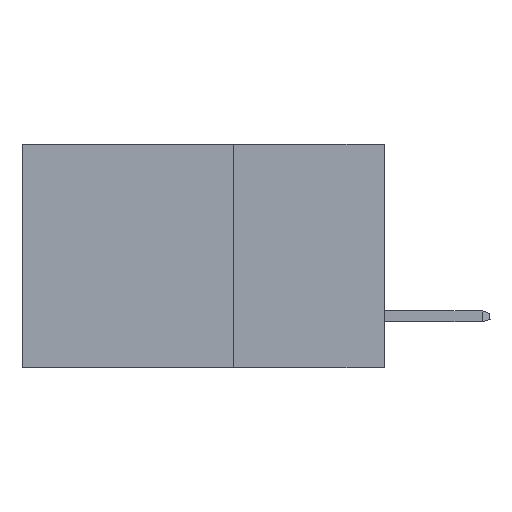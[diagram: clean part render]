
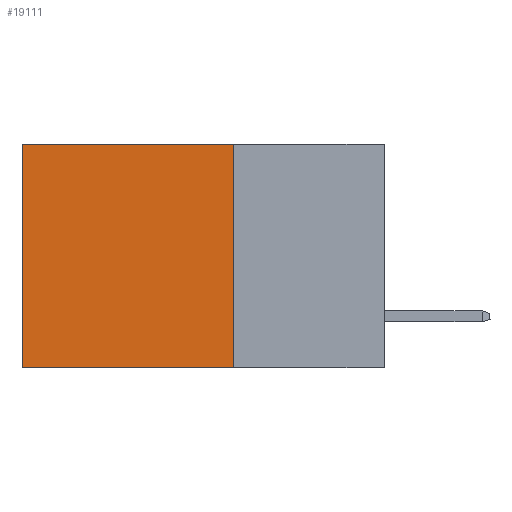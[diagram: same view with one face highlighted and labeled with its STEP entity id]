
A CAD part, left-side view. The second image highlights one B-rep face of the part: STEP entity #19111.
In plain terms, the highlighted planar face has unit normal (-1, 0, 0).
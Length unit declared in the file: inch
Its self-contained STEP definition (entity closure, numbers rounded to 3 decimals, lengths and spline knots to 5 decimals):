
#1761 = VERTEX_POINT ( 'NONE', #13774 ) ;
#2124 = EDGE_CURVE ( 'NONE', #1761, #4049, #20115, .T. ) ;
#2345 = FACE_OUTER_BOUND ( 'NONE', #21001, .T. ) ;
#3135 = AXIS2_PLACEMENT_3D ( 'NONE', #10814, #3957, #5588 ) ;
#3885 = PLANE ( 'NONE',  #3135 ) ;
#3957 = DIRECTION ( 'NONE',  ( 1., 0., 0. ) ) ;
#4049 = VERTEX_POINT ( 'NONE', #19648 ) ;
#4258 = VECTOR ( 'NONE', #10542, 39.37008 ) ;
#5027 = LINE ( 'NONE', #10880, #5830 ) ;
#5297 = CARTESIAN_POINT ( 'NONE',  ( 0.298, 0.25, -0.37 ) ) ;
#5588 = DIRECTION ( 'NONE',  ( 0., 0., -1. ) ) ;
#5607 = CARTESIAN_POINT ( 'NONE',  ( 0.298, 0.6, 0. ) ) ;
#5830 = VECTOR ( 'NONE', #12564, 39.37008 ) ;
#5952 = LINE ( 'NONE', #5297, #18921 ) ;
#8344 = CARTESIAN_POINT ( 'NONE',  ( 0.298, 0.25, 0. ) ) ;
#8613 = ORIENTED_EDGE ( 'NONE', *, *, #2124, .F. ) ;
#8927 = LINE ( 'NONE', #20661, #4258 ) ;
#10542 = DIRECTION ( 'NONE',  ( 0., 0., -1. ) ) ;
#10814 = CARTESIAN_POINT ( 'NONE',  ( 0.298, 0.25, 0. ) ) ;
#10880 = CARTESIAN_POINT ( 'NONE',  ( 0.298, 0.25, 0. ) ) ;
#11384 = ORIENTED_EDGE ( 'NONE', *, *, #20310, .F. ) ;
#12564 = DIRECTION ( 'NONE',  ( 0., 1., 0. ) ) ;
#13554 = ORIENTED_EDGE ( 'NONE', *, *, #13837, .T. ) ;
#13774 = CARTESIAN_POINT ( 'NONE',  ( 0.298, 0.25, 0. ) ) ;
#13837 = EDGE_CURVE ( 'NONE', #15859, #19630, #8927, .T. ) ;
#14537 = EDGE_CURVE ( 'NONE', #1761, #15859, #5027, .T. ) ;
#15740 = VECTOR ( 'NONE', #21278, 39.37008 ) ;
#15859 = VERTEX_POINT ( 'NONE', #5607 ) ;
#18765 = DIRECTION ( 'NONE',  ( 0., 1., 0. ) ) ;
#18921 = VECTOR ( 'NONE', #18765, 39.37008 ) ;
#19065 = CARTESIAN_POINT ( 'NONE',  ( 0.298, 0.6, -0.37 ) ) ;
#19111 = ADVANCED_FACE ( 'NONE', ( #2345 ), #3885, .F. ) ;
#19630 = VERTEX_POINT ( 'NONE', #19065 ) ;
#19648 = CARTESIAN_POINT ( 'NONE',  ( 0.298, 0.25, -0.37 ) ) ;
#20115 = LINE ( 'NONE', #8344, #15740 ) ;
#20310 = EDGE_CURVE ( 'NONE', #4049, #19630, #5952, .T. ) ;
#20661 = CARTESIAN_POINT ( 'NONE',  ( 0.298, 0.6, 0. ) ) ;
#21001 = EDGE_LOOP ( 'NONE', ( #13554, #11384, #8613, #21302 ) ) ;
#21278 = DIRECTION ( 'NONE',  ( 0., 0., -1. ) ) ;
#21302 = ORIENTED_EDGE ( 'NONE', *, *, #14537, .T. ) ;
